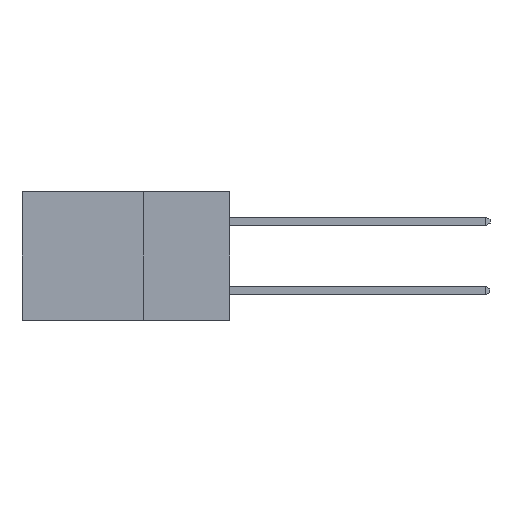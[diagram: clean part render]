
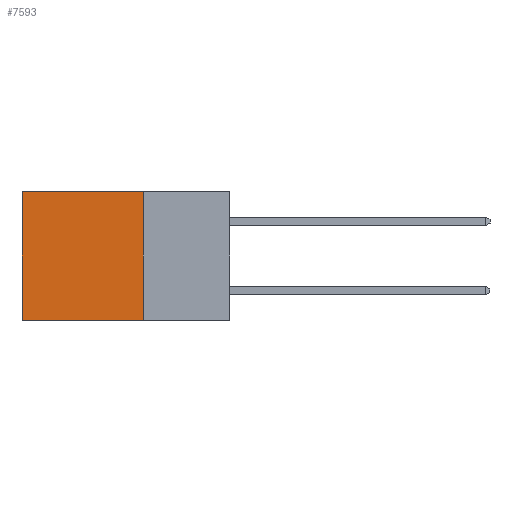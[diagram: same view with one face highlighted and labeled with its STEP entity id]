
A CAD part, left-side view. The second image highlights one B-rep face of the part: STEP entity #7593.
In plain terms, the highlighted planar face has unit normal (-1, 0, 0).
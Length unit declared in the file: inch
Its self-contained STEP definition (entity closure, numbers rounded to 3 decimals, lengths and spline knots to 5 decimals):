
#96 = EDGE_CURVE ( 'NONE', #10319, #2418, #4665, .T. ) ;
#600 = VERTEX_POINT ( 'NONE', #2888 ) ;
#1678 = CARTESIAN_POINT ( 'NONE',  ( 0.298, 0.6, 0. ) ) ;
#2418 = VERTEX_POINT ( 'NONE', #7426 ) ;
#2569 = AXIS2_PLACEMENT_3D ( 'NONE', #10887, #13189, #6439 ) ;
#2611 = VERTEX_POINT ( 'NONE', #10460 ) ;
#2888 = CARTESIAN_POINT ( 'NONE',  ( 0.298, 0.25, -0.37 ) ) ;
#3856 = LINE ( 'NONE', #4558, #10562 ) ;
#3888 = CARTESIAN_POINT ( 'NONE',  ( 0.298, 0.25, 0. ) ) ;
#4067 = ORIENTED_EDGE ( 'NONE', *, *, #5618, .F. ) ;
#4106 = ORIENTED_EDGE ( 'NONE', *, *, #8715, .T. ) ;
#4558 = CARTESIAN_POINT ( 'NONE',  ( 0.298, 0.25, -0.37 ) ) ;
#4665 = LINE ( 'NONE', #11411, #13686 ) ;
#4764 = LINE ( 'NONE', #3888, #13058 ) ;
#5618 = EDGE_CURVE ( 'NONE', #600, #2611, #3856, .T. ) ;
#5774 = FACE_OUTER_BOUND ( 'NONE', #9769, .T. ) ;
#6439 = DIRECTION ( 'NONE',  ( 0., 0., -1. ) ) ;
#7149 = ORIENTED_EDGE ( 'NONE', *, *, #96, .T. ) ;
#7426 = CARTESIAN_POINT ( 'NONE',  ( 0.298, 0.6, 0. ) ) ;
#7526 = LINE ( 'NONE', #1678, #13519 ) ;
#7593 = ADVANCED_FACE ( 'NONE', ( #5774 ), #12003, .F. ) ;
#8100 = ORIENTED_EDGE ( 'NONE', *, *, #14585, .F. ) ;
#8715 = EDGE_CURVE ( 'NONE', #2418, #2611, #7526, .T. ) ;
#9539 = CARTESIAN_POINT ( 'NONE',  ( 0.298, 0.25, 0. ) ) ;
#9711 = DIRECTION ( 'NONE',  ( 0., 0., -1. ) ) ;
#9769 = EDGE_LOOP ( 'NONE', ( #4106, #4067, #8100, #7149 ) ) ;
#10319 = VERTEX_POINT ( 'NONE', #9539 ) ;
#10460 = CARTESIAN_POINT ( 'NONE',  ( 0.298, 0.6, -0.37 ) ) ;
#10562 = VECTOR ( 'NONE', #11562, 39.37008 ) ;
#10668 = DIRECTION ( 'NONE',  ( 0., 1., 0. ) ) ;
#10887 = CARTESIAN_POINT ( 'NONE',  ( 0.298, 0.25, 0. ) ) ;
#11411 = CARTESIAN_POINT ( 'NONE',  ( 0.298, 0.25, 0. ) ) ;
#11562 = DIRECTION ( 'NONE',  ( 0., 1., 0. ) ) ;
#11755 = DIRECTION ( 'NONE',  ( 0., 0., -1. ) ) ;
#12003 = PLANE ( 'NONE',  #2569 ) ;
#13058 = VECTOR ( 'NONE', #11755, 39.37008 ) ;
#13189 = DIRECTION ( 'NONE',  ( 1., 0., 0. ) ) ;
#13519 = VECTOR ( 'NONE', #9711, 39.37008 ) ;
#13686 = VECTOR ( 'NONE', #10668, 39.37008 ) ;
#14585 = EDGE_CURVE ( 'NONE', #10319, #600, #4764, .T. ) ;
